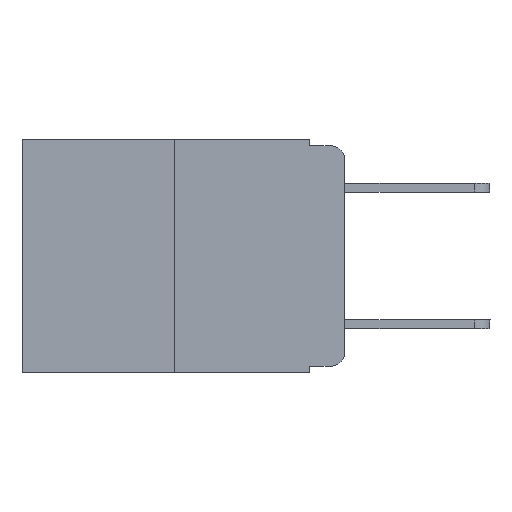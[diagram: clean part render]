
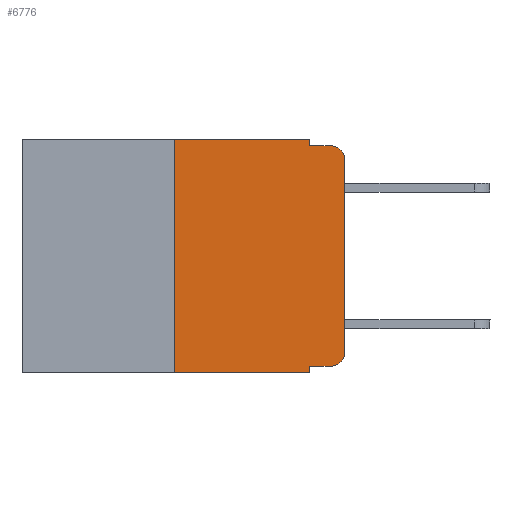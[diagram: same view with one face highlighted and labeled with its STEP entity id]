
A CAD part, left-side view. The second image highlights one B-rep face of the part: STEP entity #6776.
In plain terms, the highlighted planar face has unit normal (-1, 0, 0).
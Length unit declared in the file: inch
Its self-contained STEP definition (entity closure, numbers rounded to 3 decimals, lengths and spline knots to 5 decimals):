
#127 = DIRECTION ( 'NONE',  ( 0., 0., -1. ) ) ;
#148 = EDGE_CURVE ( 'NONE', #1645, #10874, #14077, .T. ) ;
#175 = CARTESIAN_POINT ( 'NONE',  ( 0., 0.051, -0.333 ) ) ;
#294 = ORIENTED_EDGE ( 'NONE', *, *, #14874, .F. ) ;
#339 = EDGE_CURVE ( 'NONE', #10841, #5202, #6363, .T. ) ;
#704 = ORIENTED_EDGE ( 'NONE', *, *, #11025, .F. ) ;
#806 = CARTESIAN_POINT ( 'NONE',  ( 0., 0.473, 0. ) ) ;
#1166 = ORIENTED_EDGE ( 'NONE', *, *, #148, .T. ) ;
#1285 = LINE ( 'NONE', #8181, #9180 ) ;
#1633 = VECTOR ( 'NONE', #2527, 39.37008 ) ;
#1645 = VERTEX_POINT ( 'NONE', #9536 ) ;
#1976 = AXIS2_PLACEMENT_3D ( 'NONE', #8781, #2799, #6480 ) ;
#2037 = CARTESIAN_POINT ( 'NONE',  ( 0., 0.051, -0.333 ) ) ;
#2067 = VECTOR ( 'NONE', #7881, 39.37008 ) ;
#2143 = LINE ( 'NONE', #14740, #4902 ) ;
#2163 = EDGE_LOOP ( 'NONE', ( #10831, #1166, #294, #14973, #704, #14028, #12882, #8414, #7343, #7647 ) ) ;
#2294 = LINE ( 'NONE', #4370, #5788 ) ;
#2383 = VECTOR ( 'NONE', #4402, 39.37008 ) ;
#2416 = EDGE_CURVE ( 'NONE', #4070, #5202, #8968, .T. ) ;
#2527 = DIRECTION ( 'NONE',  ( 0., -1., 0. ) ) ;
#2757 = EDGE_CURVE ( 'NONE', #12173, #12008, #10606, .T. ) ;
#2799 = DIRECTION ( 'NONE',  ( 1., 0., 0. ) ) ;
#3295 = DIRECTION ( 'NONE',  ( 0., 0., 1. ) ) ;
#3689 = CARTESIAN_POINT ( 'NONE',  ( 0., 0.25, -0.343 ) ) ;
#3797 = EDGE_CURVE ( 'NONE', #10841, #6877, #2143, .T. ) ;
#3985 = PLANE ( 'NONE',  #1976 ) ;
#4070 = VERTEX_POINT ( 'NONE', #2037 ) ;
#4366 = DIRECTION ( 'NONE',  ( -1., 0., 0. ) ) ;
#4370 = CARTESIAN_POINT ( 'NONE',  ( 0., 0., 0. ) ) ;
#4402 = DIRECTION ( 'NONE',  ( 0., 0., -1. ) ) ;
#4769 = DIRECTION ( 'NONE',  ( 0., 0., 1. ) ) ;
#4902 = VECTOR ( 'NONE', #4769, 39.37008 ) ;
#5202 = VERTEX_POINT ( 'NONE', #14090 ) ;
#5362 = FACE_OUTER_BOUND ( 'NONE', #2163, .T. ) ;
#5416 = DIRECTION ( 'NONE',  ( 0., -1., 0. ) ) ;
#5476 = VECTOR ( 'NONE', #5416, 39.37008 ) ;
#5788 = VECTOR ( 'NONE', #3295, 39.37008 ) ;
#6118 = CARTESIAN_POINT ( 'NONE',  ( 0., 0.02, -0.01 ) ) ;
#6363 = LINE ( 'NONE', #7567, #5476 ) ;
#6480 = DIRECTION ( 'NONE',  ( 0., 0., -1. ) ) ;
#6602 = CARTESIAN_POINT ( 'NONE',  ( 0., 0.02, -0.313 ) ) ;
#6776 = ADVANCED_FACE ( 'NONE', ( #5362 ), #3985, .F. ) ;
#6877 = VERTEX_POINT ( 'NONE', #11342 ) ;
#7307 = EDGE_CURVE ( 'NONE', #14835, #9201, #9932, .T. ) ;
#7343 = ORIENTED_EDGE ( 'NONE', *, *, #12000, .T. ) ;
#7380 = VECTOR ( 'NONE', #13609, 39.37008 ) ;
#7567 = CARTESIAN_POINT ( 'NONE',  ( 0., 0.473, -0.343 ) ) ;
#7647 = ORIENTED_EDGE ( 'NONE', *, *, #2757, .T. ) ;
#7881 = DIRECTION ( 'NONE',  ( 0., -1., 0. ) ) ;
#8122 = CARTESIAN_POINT ( 'NONE',  ( 0., 0.02, -0.03 ) ) ;
#8181 = CARTESIAN_POINT ( 'NONE',  ( 0., 0.051, -0.01 ) ) ;
#8414 = ORIENTED_EDGE ( 'NONE', *, *, #2416, .F. ) ;
#8781 = CARTESIAN_POINT ( 'NONE',  ( 0., 0.473, 0. ) ) ;
#8968 = LINE ( 'NONE', #9161, #2383 ) ;
#9161 = CARTESIAN_POINT ( 'NONE',  ( 0., 0.051, 0. ) ) ;
#9180 = VECTOR ( 'NONE', #9360, 39.37008 ) ;
#9201 = VERTEX_POINT ( 'NONE', #10975 ) ;
#9360 = DIRECTION ( 'NONE',  ( 0., -1., 0. ) ) ;
#9536 = CARTESIAN_POINT ( 'NONE',  ( 0., 0., -0.03 ) ) ;
#9800 = AXIS2_PLACEMENT_3D ( 'NONE', #6602, #4366, #13704 ) ;
#9932 = LINE ( 'NONE', #13556, #7380 ) ;
#10110 = EDGE_CURVE ( 'NONE', #12008, #1645, #2294, .T. ) ;
#10606 = CIRCLE ( 'NONE', #9800, 0.02 ) ;
#10831 = ORIENTED_EDGE ( 'NONE', *, *, #10110, .T. ) ;
#10841 = VERTEX_POINT ( 'NONE', #3689 ) ;
#10874 = VERTEX_POINT ( 'NONE', #6118 ) ;
#10975 = CARTESIAN_POINT ( 'NONE',  ( 0., 0.051, -0.01 ) ) ;
#11025 = EDGE_CURVE ( 'NONE', #6877, #14835, #13575, .T. ) ;
#11342 = CARTESIAN_POINT ( 'NONE',  ( 0., 0.25, 0. ) ) ;
#11883 = CARTESIAN_POINT ( 'NONE',  ( 0., 0.051, 0. ) ) ;
#12000 = EDGE_CURVE ( 'NONE', #4070, #12173, #14802, .T. ) ;
#12008 = VERTEX_POINT ( 'NONE', #14211 ) ;
#12173 = VERTEX_POINT ( 'NONE', #14390 ) ;
#12882 = ORIENTED_EDGE ( 'NONE', *, *, #339, .T. ) ;
#13016 = AXIS2_PLACEMENT_3D ( 'NONE', #8122, #13923, #127 ) ;
#13556 = CARTESIAN_POINT ( 'NONE',  ( 0., 0.051, 0. ) ) ;
#13575 = LINE ( 'NONE', #806, #2067 ) ;
#13609 = DIRECTION ( 'NONE',  ( 0., 0., -1. ) ) ;
#13704 = DIRECTION ( 'NONE',  ( 0., 0., -1. ) ) ;
#13923 = DIRECTION ( 'NONE',  ( -1., 0., 0. ) ) ;
#14028 = ORIENTED_EDGE ( 'NONE', *, *, #3797, .F. ) ;
#14077 = CIRCLE ( 'NONE', #13016, 0.02 ) ;
#14090 = CARTESIAN_POINT ( 'NONE',  ( 0., 0.051, -0.343 ) ) ;
#14211 = CARTESIAN_POINT ( 'NONE',  ( 0., 0., -0.313 ) ) ;
#14390 = CARTESIAN_POINT ( 'NONE',  ( 0., 0.02, -0.333 ) ) ;
#14740 = CARTESIAN_POINT ( 'NONE',  ( 0., 0.25, 0. ) ) ;
#14802 = LINE ( 'NONE', #175, #1633 ) ;
#14835 = VERTEX_POINT ( 'NONE', #11883 ) ;
#14874 = EDGE_CURVE ( 'NONE', #9201, #10874, #1285, .T. ) ;
#14973 = ORIENTED_EDGE ( 'NONE', *, *, #7307, .F. ) ;
